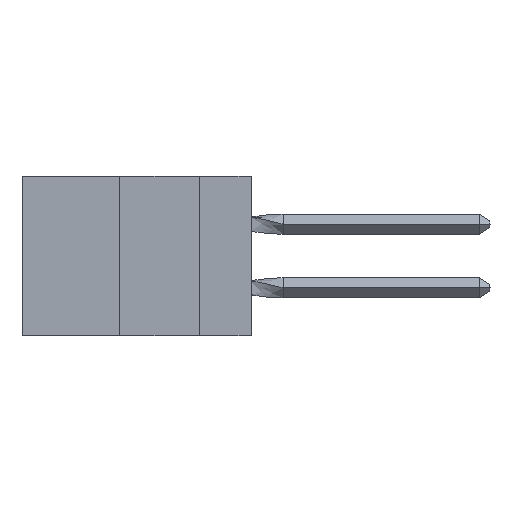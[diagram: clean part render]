
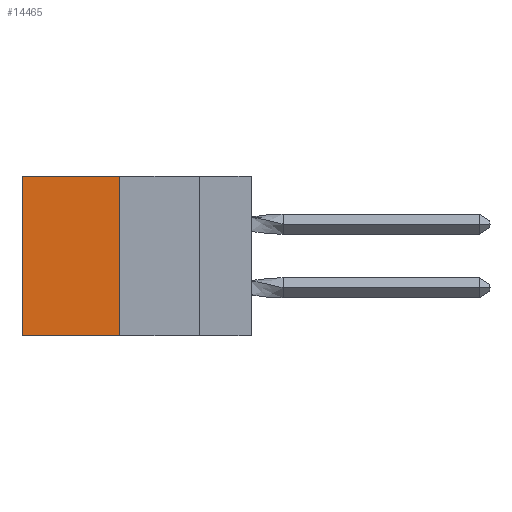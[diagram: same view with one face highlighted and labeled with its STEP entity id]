
A CAD part, left-side view. The second image highlights one B-rep face of the part: STEP entity #14465.
In plain terms, the highlighted planar face has unit normal (-1, 0, 0).
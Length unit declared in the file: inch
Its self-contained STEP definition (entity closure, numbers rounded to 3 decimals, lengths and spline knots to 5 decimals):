
#548 = CARTESIAN_POINT ( 'NONE',  ( 0.305, 0.72, -0.5 ) ) ;
#835 = ORIENTED_EDGE ( 'NONE', *, *, #3252, .F. ) ;
#1284 = VERTEX_POINT ( 'NONE', #6511 ) ;
#1779 = CARTESIAN_POINT ( 'NONE',  ( 0.305, 0.72, -0.5 ) ) ;
#2553 = CARTESIAN_POINT ( 'NONE',  ( 0.305, 0.413, -0.5 ) ) ;
#3252 = EDGE_CURVE ( 'NONE', #1284, #13165, #7477, .T. ) ;
#3987 = LINE ( 'NONE', #1779, #4429 ) ;
#4028 = DIRECTION ( 'NONE',  ( 0., 1., 0. ) ) ;
#4429 = VECTOR ( 'NONE', #16797, 39.37008 ) ;
#4665 = EDGE_CURVE ( 'NONE', #10724, #12577, #3987, .T. ) ;
#4676 = CARTESIAN_POINT ( 'NONE',  ( 0.305, 0.413, -0.5 ) ) ;
#4732 = ORIENTED_EDGE ( 'NONE', *, *, #10917, .F. ) ;
#5313 = ORIENTED_EDGE ( 'NONE', *, *, #6309, .T. ) ;
#5367 = CARTESIAN_POINT ( 'NONE',  ( 0.305, 0.413, -0.5 ) ) ;
#6150 = AXIS2_PLACEMENT_3D ( 'NONE', #5367, #13718, #8272 ) ;
#6309 = EDGE_CURVE ( 'NONE', #1284, #10724, #14581, .T. ) ;
#6511 = CARTESIAN_POINT ( 'NONE',  ( 0.305, 0.413, 0. ) ) ;
#7477 = LINE ( 'NONE', #4676, #12399 ) ;
#7855 = DIRECTION ( 'NONE',  ( 0., 0., -1. ) ) ;
#8272 = DIRECTION ( 'NONE',  ( 0., 0., -1. ) ) ;
#8573 = VECTOR ( 'NONE', #14970, 39.37008 ) ;
#8958 = CARTESIAN_POINT ( 'NONE',  ( 0.305, 0.413, -0.5 ) ) ;
#10724 = VERTEX_POINT ( 'NONE', #15939 ) ;
#10789 = LINE ( 'NONE', #2553, #16812 ) ;
#10917 = EDGE_CURVE ( 'NONE', #13165, #12577, #10789, .T. ) ;
#12225 = EDGE_LOOP ( 'NONE', ( #12332, #4732, #835, #5313 ) ) ;
#12332 = ORIENTED_EDGE ( 'NONE', *, *, #4665, .T. ) ;
#12399 = VECTOR ( 'NONE', #7855, 39.37008 ) ;
#12577 = VERTEX_POINT ( 'NONE', #548 ) ;
#13165 = VERTEX_POINT ( 'NONE', #8958 ) ;
#13718 = DIRECTION ( 'NONE',  ( 1., 0., 0. ) ) ;
#14104 = FACE_OUTER_BOUND ( 'NONE', #12225, .T. ) ;
#14465 = ADVANCED_FACE ( 'NONE', ( #14104 ), #16566, .F. ) ;
#14581 = LINE ( 'NONE', #14916, #8573 ) ;
#14916 = CARTESIAN_POINT ( 'NONE',  ( 0.305, 0.413, 0. ) ) ;
#14970 = DIRECTION ( 'NONE',  ( 0., 1., 0. ) ) ;
#15939 = CARTESIAN_POINT ( 'NONE',  ( 0.305, 0.72, 0. ) ) ;
#16566 = PLANE ( 'NONE',  #6150 ) ;
#16797 = DIRECTION ( 'NONE',  ( 0., 0., -1. ) ) ;
#16812 = VECTOR ( 'NONE', #4028, 39.37008 ) ;
